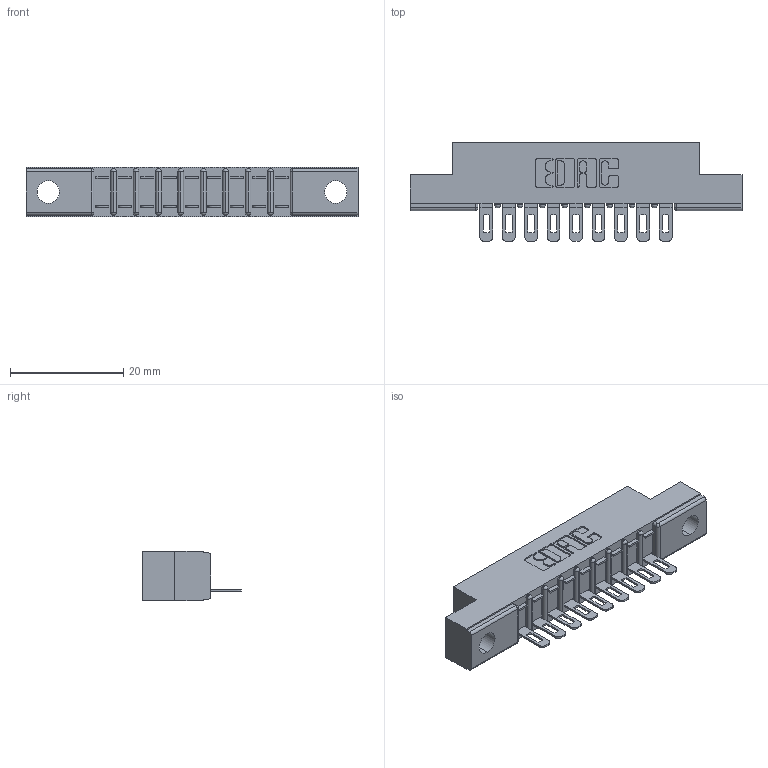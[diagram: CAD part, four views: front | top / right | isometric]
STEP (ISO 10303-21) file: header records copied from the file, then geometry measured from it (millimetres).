
FILE_DESCRIPTION (( 'STEP AP203' ), '1' );
FILE_NAME ('357-009-401-104.STEP', '2020-09-30T05:45:56', ( '' ), ( '' ), 'SwSTEP 2.0', 'SolidWorks 2020', '' );
FILE_SCHEMA (( 'CONFIG_CONTROL_DESIGN' ));
Length unit declared in the file: inch
Products named in the file (3): 307-290-002_501; 307 Part_.156 Dia Mounting Holes; 357-009-401-104
Assembly tree (10 placements, depth 2):
  357-009-401-104
    307 Part_.156 Dia Mounting Holes
    307-290-002_501  x9
Bounding box: 58.67 x 17.42 x 8.71 mm (x, y, z)
Volume: 3768.6 mm3; surface area: 6083 mm2
Topology: 10 solids, 10 shells, 826 faces, 2501 edges, 1638 vertices
Faces by surface type: plane 480, cylinder 326, sphere 20
Entity records: 12996 total; most frequent: CARTESIAN_POINT 2190, ORIENTED_EDGE 2178, DIRECTION 2139, EDGE_CURVE 1089, LINE 821, VECTOR 821, VERTEX_POINT 710, AXIS2_PLACEMENT_3D 659
